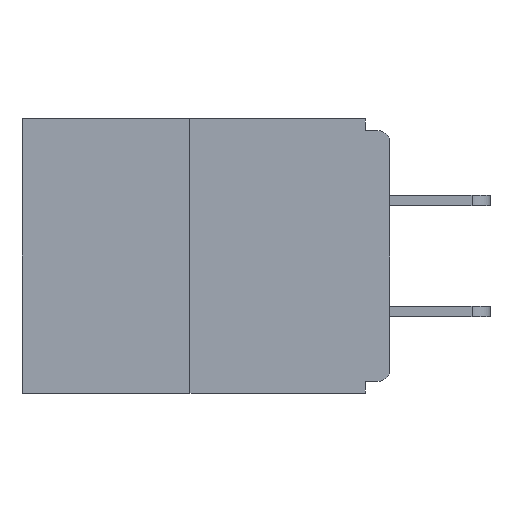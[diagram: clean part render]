
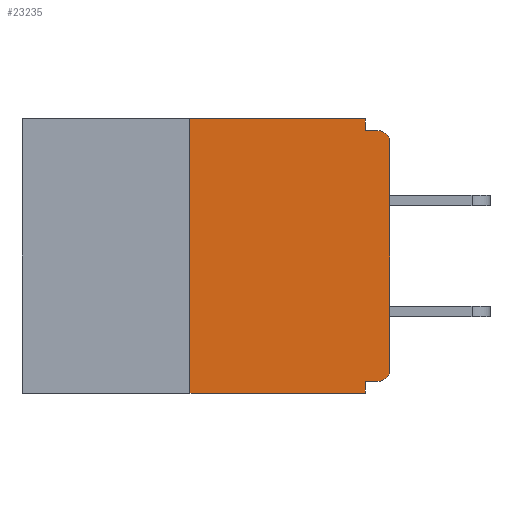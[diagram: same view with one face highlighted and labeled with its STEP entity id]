
A CAD part, left-side view. The second image highlights one B-rep face of the part: STEP entity #23235.
In plain terms, the highlighted planar face has unit normal (-1, 0, 0).
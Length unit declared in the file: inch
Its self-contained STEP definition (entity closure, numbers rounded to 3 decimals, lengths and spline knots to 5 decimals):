
#72 = DIRECTION ( 'NONE',  ( 0., 0., -1. ) ) ;
#701 = DIRECTION ( 'NONE',  ( 0., -1., 0. ) ) ;
#808 = EDGE_CURVE ( 'NONE', #17889, #5510, #8548, .T. ) ;
#838 = VECTOR ( 'NONE', #7588, 39.37008 ) ;
#1112 = CARTESIAN_POINT ( 'NONE',  ( 0., 0.015, -0.328 ) ) ;
#1361 = VECTOR ( 'NONE', #4941, 39.37008 ) ;
#1546 = VERTEX_POINT ( 'NONE', #1112 ) ;
#1842 = CARTESIAN_POINT ( 'NONE',  ( 0., 0.46, -0.343 ) ) ;
#1890 = ORIENTED_EDGE ( 'NONE', *, *, #2029, .T. ) ;
#2026 = VECTOR ( 'NONE', #20948, 39.37008 ) ;
#2029 = EDGE_CURVE ( 'NONE', #1546, #18614, #8226, .T. ) ;
#2431 = CARTESIAN_POINT ( 'NONE',  ( 0., 0., -0.03 ) ) ;
#2895 = ORIENTED_EDGE ( 'NONE', *, *, #18979, .T. ) ;
#2927 = VECTOR ( 'NONE', #23680, 39.37008 ) ;
#3184 = CARTESIAN_POINT ( 'NONE',  ( 0., 0.015, -0.313 ) ) ;
#3379 = CARTESIAN_POINT ( 'NONE',  ( 0., 0., -0.015 ) ) ;
#3773 = DIRECTION ( 'NONE',  ( 0., 0., 1. ) ) ;
#4807 = ORIENTED_EDGE ( 'NONE', *, *, #5603, .F. ) ;
#4941 = DIRECTION ( 'NONE',  ( 0., 0., 1. ) ) ;
#5327 = DIRECTION ( 'NONE',  ( 0., -1., 0. ) ) ;
#5379 = EDGE_LOOP ( 'NONE', ( #10312, #11757, #6207, #14992, #15321, #1890, #2895, #8793, #4807, #6646 ) ) ;
#5510 = VERTEX_POINT ( 'NONE', #21317 ) ;
#5603 = EDGE_CURVE ( 'NONE', #5510, #15663, #9512, .T. ) ;
#5687 = CARTESIAN_POINT ( 'NONE',  ( 0., 0.25, 0. ) ) ;
#6066 = CIRCLE ( 'NONE', #21023, 0.015 ) ;
#6207 = ORIENTED_EDGE ( 'NONE', *, *, #21873, .T. ) ;
#6646 = ORIENTED_EDGE ( 'NONE', *, *, #808, .F. ) ;
#7112 = VECTOR ( 'NONE', #13074, 39.37008 ) ;
#7588 = DIRECTION ( 'NONE',  ( 0., 1., 0. ) ) ;
#7889 = CARTESIAN_POINT ( 'NONE',  ( 0., 0., -0.328 ) ) ;
#8226 = CIRCLE ( 'NONE', #17455, 0.015 ) ;
#8548 = LINE ( 'NONE', #9245, #7112 ) ;
#8793 = ORIENTED_EDGE ( 'NONE', *, *, #11251, .T. ) ;
#9245 = CARTESIAN_POINT ( 'NONE',  ( 0., 0.031, 0. ) ) ;
#9493 = AXIS2_PLACEMENT_3D ( 'NONE', #18492, #14633, #72 ) ;
#9512 = LINE ( 'NONE', #3379, #2927 ) ;
#9847 = CARTESIAN_POINT ( 'NONE',  ( 0., 0.031, -0.328 ) ) ;
#9930 = LINE ( 'NONE', #18038, #1361 ) ;
#10011 = LINE ( 'NONE', #19024, #2026 ) ;
#10278 = CARTESIAN_POINT ( 'NONE',  ( 0., 0.031, -0.343 ) ) ;
#10312 = ORIENTED_EDGE ( 'NONE', *, *, #20481, .F. ) ;
#11251 = EDGE_CURVE ( 'NONE', #19503, #15663, #6066, .T. ) ;
#11687 = CARTESIAN_POINT ( 'NONE',  ( 0., 0.25, -0.343 ) ) ;
#11757 = ORIENTED_EDGE ( 'NONE', *, *, #16152, .F. ) ;
#11795 = VERTEX_POINT ( 'NONE', #5687 ) ;
#11798 = CARTESIAN_POINT ( 'NONE',  ( 0., 0., -0.313 ) ) ;
#11876 = VERTEX_POINT ( 'NONE', #9847 ) ;
#11985 = VERTEX_POINT ( 'NONE', #11687 ) ;
#13074 = DIRECTION ( 'NONE',  ( 0., 0., -1. ) ) ;
#13847 = CARTESIAN_POINT ( 'NONE',  ( 0., 0.015, -0.03 ) ) ;
#14633 = DIRECTION ( 'NONE',  ( 1., 0., 0. ) ) ;
#14788 = EDGE_CURVE ( 'NONE', #1546, #11876, #15149, .T. ) ;
#14962 = VECTOR ( 'NONE', #3773, 39.37008 ) ;
#14992 = ORIENTED_EDGE ( 'NONE', *, *, #23489, .F. ) ;
#15149 = LINE ( 'NONE', #7889, #838 ) ;
#15321 = ORIENTED_EDGE ( 'NONE', *, *, #14788, .F. ) ;
#15442 = CARTESIAN_POINT ( 'NONE',  ( 0., 0.46, 0. ) ) ;
#15663 = VERTEX_POINT ( 'NONE', #18225 ) ;
#15769 = VECTOR ( 'NONE', #701, 39.37008 ) ;
#15809 = DIRECTION ( 'NONE',  ( -1., 0., 0. ) ) ;
#16001 = DIRECTION ( 'NONE',  ( -1., 0., 0. ) ) ;
#16152 = EDGE_CURVE ( 'NONE', #11985, #11795, #9930, .T. ) ;
#16471 = PLANE ( 'NONE',  #9493 ) ;
#16514 = CARTESIAN_POINT ( 'NONE',  ( 0., 0., 0. ) ) ;
#17455 = AXIS2_PLACEMENT_3D ( 'NONE', #3184, #16001, #17850 ) ;
#17561 = DIRECTION ( 'NONE',  ( 0., 0., -1. ) ) ;
#17850 = DIRECTION ( 'NONE',  ( 0., 0., -1. ) ) ;
#17889 = VERTEX_POINT ( 'NONE', #20060 ) ;
#18038 = CARTESIAN_POINT ( 'NONE',  ( 0., 0.25, 0. ) ) ;
#18225 = CARTESIAN_POINT ( 'NONE',  ( 0., 0.015, -0.015 ) ) ;
#18492 = CARTESIAN_POINT ( 'NONE',  ( 0., 0.46, 0. ) ) ;
#18614 = VERTEX_POINT ( 'NONE', #11798 ) ;
#18979 = EDGE_CURVE ( 'NONE', #18614, #19503, #22414, .T. ) ;
#19024 = CARTESIAN_POINT ( 'NONE',  ( 0., 0.031, -0.343 ) ) ;
#19503 = VERTEX_POINT ( 'NONE', #2431 ) ;
#19590 = VERTEX_POINT ( 'NONE', #10278 ) ;
#19699 = LINE ( 'NONE', #1842, #20566 ) ;
#20060 = CARTESIAN_POINT ( 'NONE',  ( 0., 0.031, 0. ) ) ;
#20481 = EDGE_CURVE ( 'NONE', #11795, #17889, #20634, .T. ) ;
#20566 = VECTOR ( 'NONE', #5327, 39.37008 ) ;
#20634 = LINE ( 'NONE', #15442, #15769 ) ;
#20948 = DIRECTION ( 'NONE',  ( 0., 0., -1. ) ) ;
#21023 = AXIS2_PLACEMENT_3D ( 'NONE', #13847, #15809, #17561 ) ;
#21317 = CARTESIAN_POINT ( 'NONE',  ( 0., 0.031, -0.015 ) ) ;
#21506 = FACE_OUTER_BOUND ( 'NONE', #5379, .T. ) ;
#21873 = EDGE_CURVE ( 'NONE', #11985, #19590, #19699, .T. ) ;
#22414 = LINE ( 'NONE', #16514, #14962 ) ;
#23235 = ADVANCED_FACE ( 'NONE', ( #21506 ), #16471, .F. ) ;
#23489 = EDGE_CURVE ( 'NONE', #11876, #19590, #10011, .T. ) ;
#23680 = DIRECTION ( 'NONE',  ( 0., -1., 0. ) ) ;
